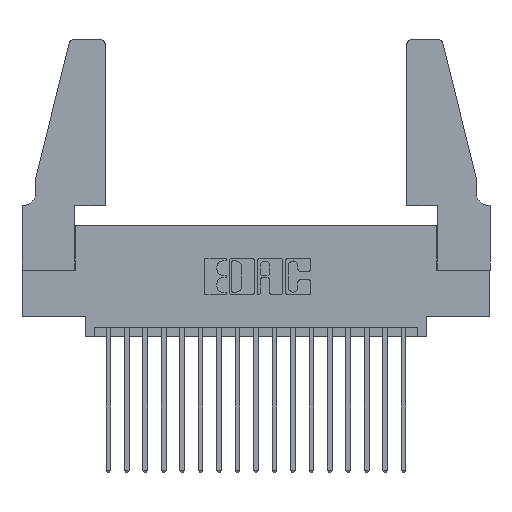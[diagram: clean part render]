
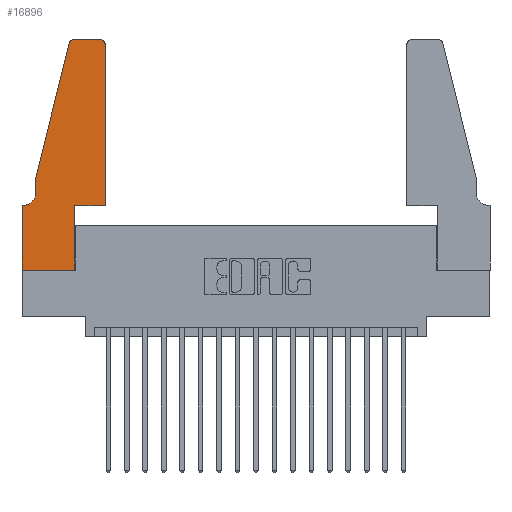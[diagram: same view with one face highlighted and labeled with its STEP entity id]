
A CAD part, top view. The second image highlights one B-rep face of the part: STEP entity #16896.
In plain terms, the highlighted planar face has unit normal (0, 0, 1).
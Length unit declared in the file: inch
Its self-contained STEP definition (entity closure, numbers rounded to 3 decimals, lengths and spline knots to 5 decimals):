
#50 = VERTEX_POINT ( 'NONE', #4194 ) ;
#152 = VERTEX_POINT ( 'NONE', #18236 ) ;
#475 = VERTEX_POINT ( 'NONE', #5075 ) ;
#799 = EDGE_LOOP ( 'NONE', ( #5018, #12221, #4435, #9655, #11912, #11020, #5630, #6683, #8423, #2843, #10764, #18197 ) ) ;
#826 = CIRCLE ( 'NONE', #15149, 0.03 ) ;
#975 = DIRECTION ( 'NONE',  ( 1., 0., 0. ) ) ;
#1069 = FACE_OUTER_BOUND ( 'NONE', #799, .T. ) ;
#1090 = EDGE_CURVE ( 'NONE', #4660, #13023, #826, .T. ) ;
#2441 = DIRECTION ( 'NONE',  ( -1., 0., 0. ) ) ;
#2519 = VECTOR ( 'NONE', #8190, 39.37008 ) ;
#2820 = AXIS2_PLACEMENT_3D ( 'NONE', #5003, #15296, #6532 ) ;
#2843 = ORIENTED_EDGE ( 'NONE', *, *, #18022, .T. ) ;
#3622 = CARTESIAN_POINT ( 'NONE',  ( 0.2865, 0.35, 0.37 ) ) ;
#3815 = DIRECTION ( 'NONE',  ( 0., 0., 1. ) ) ;
#3968 = CARTESIAN_POINT ( 'NONE',  ( 0.4505, 0.35, 0.37 ) ) ;
#4132 = VERTEX_POINT ( 'NONE', #17924 ) ;
#4194 = CARTESIAN_POINT ( 'NONE',  ( 0.2865, 0., 0.37 ) ) ;
#4219 = CARTESIAN_POINT ( 'NONE',  ( 0., 0.35, 0.37 ) ) ;
#4432 = CARTESIAN_POINT ( 'NONE',  ( 0., 0., 0.37 ) ) ;
#4435 = ORIENTED_EDGE ( 'NONE', *, *, #17900, .T. ) ;
#4660 = VERTEX_POINT ( 'NONE', #12205 ) ;
#5003 = CARTESIAN_POINT ( 'NONE',  ( 0.0055, 0.42, 0.37 ) ) ;
#5018 = ORIENTED_EDGE ( 'NONE', *, *, #16763, .T. ) ;
#5075 = CARTESIAN_POINT ( 'NONE',  ( 0.0055, 0.35, 0.37 ) ) ;
#5131 = VERTEX_POINT ( 'NONE', #4219 ) ;
#5178 = VECTOR ( 'NONE', #16802, 39.37008 ) ;
#5205 = LINE ( 'NONE', #10521, #13539 ) ;
#5323 = CARTESIAN_POINT ( 'NONE',  ( 0.0755, 0.5, 0.37 ) ) ;
#5562 = VERTEX_POINT ( 'NONE', #15490 ) ;
#5630 = ORIENTED_EDGE ( 'NONE', *, *, #11060, .T. ) ;
#5663 = LINE ( 'NONE', #6644, #5178 ) ;
#5988 = EDGE_CURVE ( 'NONE', #475, #5131, #8891, .T. ) ;
#6471 = VECTOR ( 'NONE', #11633, 39.37008 ) ;
#6532 = DIRECTION ( 'NONE',  ( -1., 0., 0. ) ) ;
#6580 = LINE ( 'NONE', #3622, #2519 ) ;
#6644 = CARTESIAN_POINT ( 'NONE',  ( 0., 0., 0.37 ) ) ;
#6683 = ORIENTED_EDGE ( 'NONE', *, *, #14689, .T. ) ;
#6908 = EDGE_CURVE ( 'NONE', #4132, #14433, #5205, .T. ) ;
#6992 = PLANE ( 'NONE',  #15790 ) ;
#7048 = CARTESIAN_POINT ( 'NONE',  ( 0.0755, 0.35, 0.37 ) ) ;
#7872 = VERTEX_POINT ( 'NONE', #18267 ) ;
#7912 = LINE ( 'NONE', #8141, #14320 ) ;
#8023 = CARTESIAN_POINT ( 'NONE',  ( 0.4505, 1.22, 0.37 ) ) ;
#8141 = CARTESIAN_POINT ( 'NONE',  ( 0.2605, 1.25, 0.37 ) ) ;
#8190 = DIRECTION ( 'NONE',  ( 0., 1., 0. ) ) ;
#8423 = ORIENTED_EDGE ( 'NONE', *, *, #15465, .T. ) ;
#8477 = CARTESIAN_POINT ( 'NONE',  ( 0., 0.35, 0.37 ) ) ;
#8891 = LINE ( 'NONE', #7048, #16589 ) ;
#8976 = DIRECTION ( 'NONE',  ( 0., -1., 0. ) ) ;
#9655 = ORIENTED_EDGE ( 'NONE', *, *, #6908, .T. ) ;
#9991 = DIRECTION ( 'NONE',  ( 0., 0., 1. ) ) ;
#10187 = CARTESIAN_POINT ( 'NONE',  ( 0.4505, 0.35, 0.37 ) ) ;
#10521 = CARTESIAN_POINT ( 'NONE',  ( 0.0755, 0.5, 0.37 ) ) ;
#10764 = ORIENTED_EDGE ( 'NONE', *, *, #18067, .T. ) ;
#10900 = EDGE_CURVE ( 'NONE', #12123, #152, #17833, .T. ) ;
#10920 = VECTOR ( 'NONE', #8976, 39.37008 ) ;
#11020 = ORIENTED_EDGE ( 'NONE', *, *, #5988, .T. ) ;
#11060 = EDGE_CURVE ( 'NONE', #5131, #7872, #11360, .T. ) ;
#11327 = LINE ( 'NONE', #3968, #18463 ) ;
#11360 = LINE ( 'NONE', #4432, #10920 ) ;
#11570 = DIRECTION ( 'NONE',  ( 1., 0., 0. ) ) ;
#11633 = DIRECTION ( 'NONE',  ( 0., 1., 0. ) ) ;
#11912 = ORIENTED_EDGE ( 'NONE', *, *, #12117, .T. ) ;
#11981 = DIRECTION ( 'NONE',  ( 0., -1., 0. ) ) ;
#12117 = EDGE_CURVE ( 'NONE', #14433, #475, #15835, .T. ) ;
#12123 = VERTEX_POINT ( 'NONE', #8023 ) ;
#12205 = CARTESIAN_POINT ( 'NONE',  ( 0.284, 1.25, 0.37 ) ) ;
#12221 = ORIENTED_EDGE ( 'NONE', *, *, #1090, .T. ) ;
#12702 = DIRECTION ( 'NONE',  ( -0.239, -0.971, 0. ) ) ;
#12751 = CARTESIAN_POINT ( 'NONE',  ( 0.4205, 1.22, 0.37 ) ) ;
#13023 = VERTEX_POINT ( 'NONE', #14259 ) ;
#13539 = VECTOR ( 'NONE', #11981, 39.37008 ) ;
#14047 = LINE ( 'NONE', #5323, #16919 ) ;
#14210 = DIRECTION ( 'NONE',  ( 1., 0., 0. ) ) ;
#14259 = CARTESIAN_POINT ( 'NONE',  ( 0.25487, 1.22718, 0.37 ) ) ;
#14320 = VECTOR ( 'NONE', #16825, 39.37008 ) ;
#14433 = VERTEX_POINT ( 'NONE', #19003 ) ;
#14689 = EDGE_CURVE ( 'NONE', #7872, #50, #5663, .T. ) ;
#15149 = AXIS2_PLACEMENT_3D ( 'NONE', #16235, #18491, #16372 ) ;
#15296 = DIRECTION ( 'NONE',  ( 0., 0., -1. ) ) ;
#15465 = EDGE_CURVE ( 'NONE', #50, #15931, #6580, .T. ) ;
#15490 = CARTESIAN_POINT ( 'NONE',  ( 0.4505, 0.35, 0.37 ) ) ;
#15790 = AXIS2_PLACEMENT_3D ( 'NONE', #8477, #9991, #975 ) ;
#15835 = CIRCLE ( 'NONE', #2820, 0.07 ) ;
#15931 = VERTEX_POINT ( 'NONE', #17828 ) ;
#16180 = AXIS2_PLACEMENT_3D ( 'NONE', #12751, #3815, #14210 ) ;
#16235 = CARTESIAN_POINT ( 'NONE',  ( 0.284, 1.22, 0.37 ) ) ;
#16372 = DIRECTION ( 'NONE',  ( 1., 0., 0. ) ) ;
#16589 = VECTOR ( 'NONE', #2441, 39.37008 ) ;
#16763 = EDGE_CURVE ( 'NONE', #152, #4660, #7912, .T. ) ;
#16802 = DIRECTION ( 'NONE',  ( 1., 0., 0. ) ) ;
#16825 = DIRECTION ( 'NONE',  ( -1., 0., 0. ) ) ;
#16896 = ADVANCED_FACE ( 'NONE', ( #1069 ), #6992, .T. ) ;
#16919 = VECTOR ( 'NONE', #12702, 39.37008 ) ;
#17828 = CARTESIAN_POINT ( 'NONE',  ( 0.2865, 0.35, 0.37 ) ) ;
#17833 = CIRCLE ( 'NONE', #16180, 0.03 ) ;
#17900 = EDGE_CURVE ( 'NONE', #13023, #4132, #14047, .T. ) ;
#17924 = CARTESIAN_POINT ( 'NONE',  ( 0.0755, 0.5, 0.37 ) ) ;
#18018 = LINE ( 'NONE', #10187, #6471 ) ;
#18022 = EDGE_CURVE ( 'NONE', #15931, #5562, #11327, .T. ) ;
#18067 = EDGE_CURVE ( 'NONE', #5562, #12123, #18018, .T. ) ;
#18197 = ORIENTED_EDGE ( 'NONE', *, *, #10900, .T. ) ;
#18236 = CARTESIAN_POINT ( 'NONE',  ( 0.4205, 1.25, 0.37 ) ) ;
#18267 = CARTESIAN_POINT ( 'NONE',  ( 0., 0., 0.37 ) ) ;
#18463 = VECTOR ( 'NONE', #11570, 39.37008 ) ;
#18491 = DIRECTION ( 'NONE',  ( 0., 0., 1. ) ) ;
#19003 = CARTESIAN_POINT ( 'NONE',  ( 0.0755, 0.42, 0.37 ) ) ;
